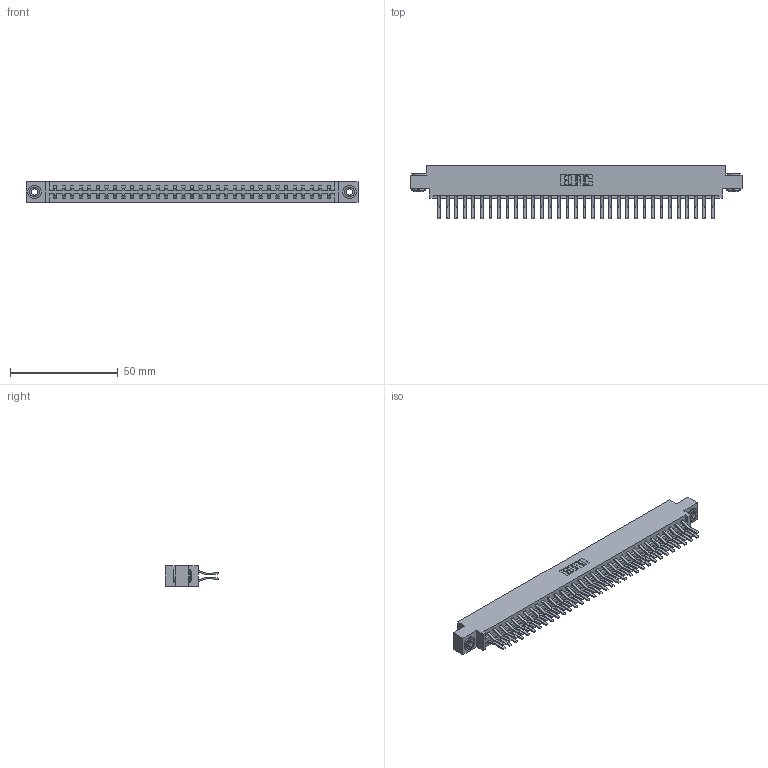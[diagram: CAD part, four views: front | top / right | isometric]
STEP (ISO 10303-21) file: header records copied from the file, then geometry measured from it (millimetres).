
FILE_DESCRIPTION (( 'STEP AP203' ), '1' );
FILE_NAME ('337-066-560-803.STEP', '2019-10-12T01:34:54', ( '' ), ( '' ), 'SwSTEP 2.0', 'SolidWorks 2016', '' );
FILE_SCHEMA (( 'CONFIG_CONTROL_DESIGN' ));
Length unit declared in the file: inch
Products named in the file (4): 345-250-002_345-250-002-102; 337-066-560-803; 337 Part_0.170 Offset - 0.156 Dia-TH; 345-292-001_560 Tail
Assembly tree (69 placements, depth 2):
  337-066-560-803
    337 Part_0.170 Offset - 0.156 Dia-TH
    345-292-001_560 Tail  x66
    345-250-002_345-250-002-102  x2
Bounding box: 153.77 x 24.78 x 9.4 mm (x, y, z)
Volume: 16420.4 mm3; surface area: 20060.1 mm2
Topology: 69 solids, 69 shells, 3852 faces, 11421 edges, 7522 vertices
Faces by surface type: plane 2592, cylinder 1252, cone 8
Entity records: 27620 total; most frequent: CARTESIAN_POINT 4637, ORIENTED_EDGE 4566, DIRECTION 3997, EDGE_CURVE 2283, VECTOR 2127, LINE 2127, VERTEX_POINT 1518, AXIS2_PLACEMENT_3D 935
